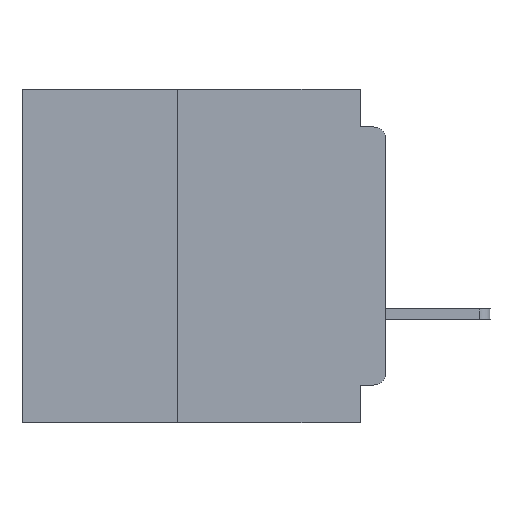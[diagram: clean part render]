
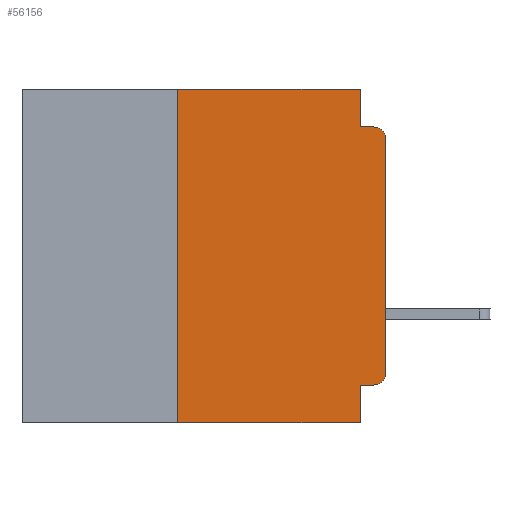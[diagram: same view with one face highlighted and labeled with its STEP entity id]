
A CAD part, left-side view. The second image highlights one B-rep face of the part: STEP entity #56156.
In plain terms, the highlighted planar face has unit normal (-1, 0, 0).
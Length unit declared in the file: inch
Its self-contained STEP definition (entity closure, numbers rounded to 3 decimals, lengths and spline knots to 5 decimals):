
#636 = EDGE_LOOP ( 'NONE', ( #57983, #12238, #14910, #8028, #25946, #54099, #23412, #39154, #44144, #47771 ) ) ;
#1113 = DIRECTION ( 'NONE',  ( 0., -1., 0. ) ) ;
#1209 = FACE_OUTER_BOUND ( 'NONE', #636, .T. ) ;
#1909 = DIRECTION ( 'NONE',  ( -1., 0., 0. ) ) ;
#2343 = EDGE_CURVE ( 'NONE', #37819, #45798, #6046, .T. ) ;
#3989 = CARTESIAN_POINT ( 'NONE',  ( 0., 0.031, -0.045 ) ) ;
#5933 = VECTOR ( 'NONE', #31384, 39.37008 ) ;
#5939 = VERTEX_POINT ( 'NONE', #13836 ) ;
#6046 = LINE ( 'NONE', #51277, #39778 ) ;
#6581 = VERTEX_POINT ( 'NONE', #52665 ) ;
#7006 = CARTESIAN_POINT ( 'NONE',  ( 0., 0.015, -0.045 ) ) ;
#7327 = PLANE ( 'NONE',  #30808 ) ;
#8028 = ORIENTED_EDGE ( 'NONE', *, *, #26854, .F. ) ;
#8673 = EDGE_CURVE ( 'NONE', #43605, #6581, #38868, .T. ) ;
#9025 = EDGE_CURVE ( 'NONE', #31490, #52823, #44419, .T. ) ;
#10267 = AXIS2_PLACEMENT_3D ( 'NONE', #43034, #16280, #47536 ) ;
#10341 = VECTOR ( 'NONE', #27940, 39.37008 ) ;
#10414 = CARTESIAN_POINT ( 'NONE',  ( 0., 0., 0. ) ) ;
#12107 = LINE ( 'NONE', #51050, #46414 ) ;
#12238 = ORIENTED_EDGE ( 'NONE', *, *, #9025, .T. ) ;
#13836 = CARTESIAN_POINT ( 'NONE',  ( 0., 0.25, 0. ) ) ;
#14910 = ORIENTED_EDGE ( 'NONE', *, *, #44264, .F. ) ;
#14963 = DIRECTION ( 'NONE',  ( 0., 0., 1. ) ) ;
#15186 = CARTESIAN_POINT ( 'NONE',  ( 0., 0., -0.34 ) ) ;
#15448 = CARTESIAN_POINT ( 'NONE',  ( 0., 0., -0.06 ) ) ;
#15713 = EDGE_CURVE ( 'NONE', #37819, #43111, #18345, .T. ) ;
#16043 = LINE ( 'NONE', #23527, #38417 ) ;
#16280 = DIRECTION ( 'NONE',  ( -1., 0., 0. ) ) ;
#16892 = CARTESIAN_POINT ( 'NONE',  ( 0., 0.031, 0. ) ) ;
#17464 = EDGE_CURVE ( 'NONE', #5939, #48933, #18919, .T. ) ;
#18345 = CIRCLE ( 'NONE', #32659, 0.015 ) ;
#18780 = LINE ( 'NONE', #45340, #52982 ) ;
#18919 = LINE ( 'NONE', #45814, #21749 ) ;
#21749 = VECTOR ( 'NONE', #27846, 39.37008 ) ;
#22353 = LINE ( 'NONE', #23510, #10341 ) ;
#23111 = VERTEX_POINT ( 'NONE', #3989 ) ;
#23412 = ORIENTED_EDGE ( 'NONE', *, *, #8673, .T. ) ;
#23510 = CARTESIAN_POINT ( 'NONE',  ( 0., 0.031, 0. ) ) ;
#23527 = CARTESIAN_POINT ( 'NONE',  ( 0., 0., -0.045 ) ) ;
#25400 = CARTESIAN_POINT ( 'NONE',  ( 0., 0.437, 0. ) ) ;
#25946 = ORIENTED_EDGE ( 'NONE', *, *, #17464, .F. ) ;
#26854 = EDGE_CURVE ( 'NONE', #48933, #23111, #22353, .T. ) ;
#27372 = DIRECTION ( 'NONE',  ( 0., 0., -1. ) ) ;
#27846 = DIRECTION ( 'NONE',  ( 0., -1., 0. ) ) ;
#27940 = DIRECTION ( 'NONE',  ( 0., 0., -1. ) ) ;
#28760 = CARTESIAN_POINT ( 'NONE',  ( 0., 0.015, -0.34 ) ) ;
#29877 = DIRECTION ( 'NONE',  ( 0., 0., -1. ) ) ;
#30735 = VECTOR ( 'NONE', #14963, 39.37008 ) ;
#30808 = AXIS2_PLACEMENT_3D ( 'NONE', #25400, #56576, #29877 ) ;
#31384 = DIRECTION ( 'NONE',  ( 0., -1., 0. ) ) ;
#31490 = VERTEX_POINT ( 'NONE', #15448 ) ;
#32126 = LINE ( 'NONE', #10414, #30735 ) ;
#32659 = AXIS2_PLACEMENT_3D ( 'NONE', #28760, #1909, #33228 ) ;
#33226 = EDGE_CURVE ( 'NONE', #45798, #6581, #18780, .T. ) ;
#33228 = DIRECTION ( 'NONE',  ( 0., 0., -1. ) ) ;
#36116 = CARTESIAN_POINT ( 'NONE',  ( 0., 0.015, -0.355 ) ) ;
#36330 = EDGE_CURVE ( 'NONE', #43605, #5939, #12107, .T. ) ;
#37786 = DIRECTION ( 'NONE',  ( 0., 0., 1. ) ) ;
#37819 = VERTEX_POINT ( 'NONE', #36116 ) ;
#38417 = VECTOR ( 'NONE', #1113, 39.37008 ) ;
#38868 = LINE ( 'NONE', #49346, #5933 ) ;
#39154 = ORIENTED_EDGE ( 'NONE', *, *, #33226, .F. ) ;
#39778 = VECTOR ( 'NONE', #50898, 39.37008 ) ;
#43034 = CARTESIAN_POINT ( 'NONE',  ( 0., 0.015, -0.06 ) ) ;
#43111 = VERTEX_POINT ( 'NONE', #15186 ) ;
#43605 = VERTEX_POINT ( 'NONE', #45613 ) ;
#44144 = ORIENTED_EDGE ( 'NONE', *, *, #2343, .F. ) ;
#44264 = EDGE_CURVE ( 'NONE', #23111, #52823, #16043, .T. ) ;
#44419 = CIRCLE ( 'NONE', #10267, 0.015 ) ;
#45340 = CARTESIAN_POINT ( 'NONE',  ( 0., 0.031, -0.4 ) ) ;
#45613 = CARTESIAN_POINT ( 'NONE',  ( 0., 0.25, -0.4 ) ) ;
#45798 = VERTEX_POINT ( 'NONE', #54391 ) ;
#45814 = CARTESIAN_POINT ( 'NONE',  ( 0., 0.437, 0. ) ) ;
#46414 = VECTOR ( 'NONE', #37786, 39.37008 ) ;
#47536 = DIRECTION ( 'NONE',  ( 0., 0., -1. ) ) ;
#47771 = ORIENTED_EDGE ( 'NONE', *, *, #15713, .T. ) ;
#48933 = VERTEX_POINT ( 'NONE', #16892 ) ;
#49346 = CARTESIAN_POINT ( 'NONE',  ( 0., 0.437, -0.4 ) ) ;
#50898 = DIRECTION ( 'NONE',  ( 0., 1., 0. ) ) ;
#51050 = CARTESIAN_POINT ( 'NONE',  ( 0., 0.25, -0.4 ) ) ;
#51277 = CARTESIAN_POINT ( 'NONE',  ( 0., 0., -0.355 ) ) ;
#52095 = EDGE_CURVE ( 'NONE', #43111, #31490, #32126, .T. ) ;
#52665 = CARTESIAN_POINT ( 'NONE',  ( 0., 0.031, -0.4 ) ) ;
#52823 = VERTEX_POINT ( 'NONE', #7006 ) ;
#52982 = VECTOR ( 'NONE', #27372, 39.37008 ) ;
#54099 = ORIENTED_EDGE ( 'NONE', *, *, #36330, .F. ) ;
#54391 = CARTESIAN_POINT ( 'NONE',  ( 0., 0.031, -0.355 ) ) ;
#56156 = ADVANCED_FACE ( 'NONE', ( #1209 ), #7327, .F. ) ;
#56576 = DIRECTION ( 'NONE',  ( 1., 0., 0. ) ) ;
#57983 = ORIENTED_EDGE ( 'NONE', *, *, #52095, .T. ) ;
